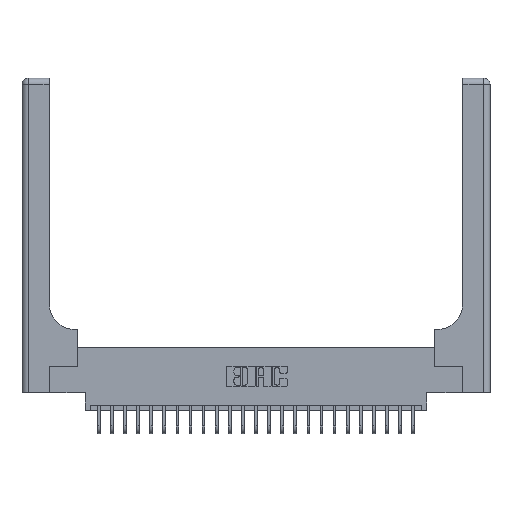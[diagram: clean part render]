
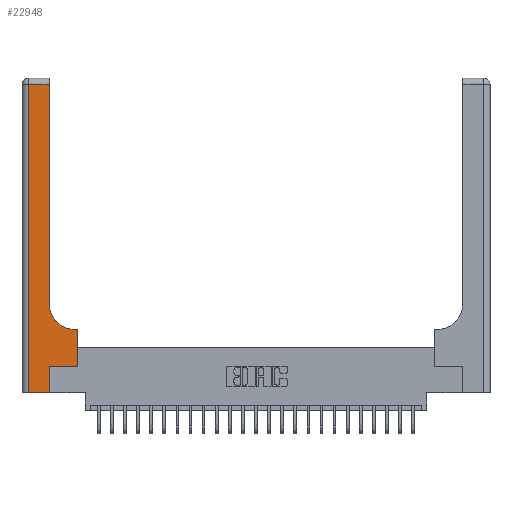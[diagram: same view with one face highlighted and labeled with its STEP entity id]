
A CAD part, top view. The second image highlights one B-rep face of the part: STEP entity #22948.
In plain terms, the highlighted planar face has unit normal (0, 0, 1).
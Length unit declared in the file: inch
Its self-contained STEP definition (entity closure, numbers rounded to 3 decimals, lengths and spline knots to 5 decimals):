
#77 = LINE ( 'NONE', #7890, #7603 ) ;
#112 = VERTEX_POINT ( 'NONE', #7689 ) ;
#280 = LINE ( 'NONE', #24262, #21089 ) ;
#475 = VERTEX_POINT ( 'NONE', #2131 ) ;
#609 = EDGE_CURVE ( 'NONE', #1662, #475, #941, .T. ) ;
#678 = CARTESIAN_POINT ( 'NONE',  ( 0.265, 0., 0.37 ) ) ;
#730 = CARTESIAN_POINT ( 'NONE',  ( 0.265, 0.25, 0.37 ) ) ;
#839 = ORIENTED_EDGE ( 'NONE', *, *, #14893, .T. ) ;
#941 = LINE ( 'NONE', #4898, #4275 ) ;
#1059 = CARTESIAN_POINT ( 'NONE',  ( 0.26, 0.6, 0.37 ) ) ;
#1343 = AXIS2_PLACEMENT_3D ( 'NONE', #14839, #16431, #24529 ) ;
#1346 = CARTESIAN_POINT ( 'NONE',  ( 0.26, 3., 0.37 ) ) ;
#1662 = VERTEX_POINT ( 'NONE', #21528 ) ;
#1991 = LINE ( 'NONE', #23966, #20015 ) ;
#2131 = CARTESIAN_POINT ( 'NONE',  ( 0.06, 2.94, 0.37 ) ) ;
#2136 = VERTEX_POINT ( 'NONE', #11423 ) ;
#3370 = AXIS2_PLACEMENT_3D ( 'NONE', #18715, #4401, #20845 ) ;
#4101 = DIRECTION ( 'NONE',  ( 0., -1., 0. ) ) ;
#4275 = VECTOR ( 'NONE', #23180, 39.37008 ) ;
#4401 = DIRECTION ( 'NONE',  ( 0., 0., -1. ) ) ;
#4898 = CARTESIAN_POINT ( 'NONE',  ( 0., 2.94, 0.37 ) ) ;
#5869 = VERTEX_POINT ( 'NONE', #25117 ) ;
#6235 = EDGE_CURVE ( 'NONE', #13222, #14108, #9724, .T. ) ;
#6571 = VERTEX_POINT ( 'NONE', #7796 ) ;
#7153 = ORIENTED_EDGE ( 'NONE', *, *, #11031, .T. ) ;
#7275 = ORIENTED_EDGE ( 'NONE', *, *, #19658, .T. ) ;
#7603 = VECTOR ( 'NONE', #16080, 39.37008 ) ;
#7689 = CARTESIAN_POINT ( 'NONE',  ( 0.528, 0.6, 0.37 ) ) ;
#7796 = CARTESIAN_POINT ( 'NONE',  ( 0.26, 0.85, 0.37 ) ) ;
#7890 = CARTESIAN_POINT ( 'NONE',  ( 0., 0., 0.37 ) ) ;
#8899 = VECTOR ( 'NONE', #13922, 39.37008 ) ;
#9143 = ORIENTED_EDGE ( 'NONE', *, *, #12044, .T. ) ;
#9724 = LINE ( 'NONE', #15902, #8899 ) ;
#10054 = ORIENTED_EDGE ( 'NONE', *, *, #25425, .T. ) ;
#11031 = EDGE_CURVE ( 'NONE', #14108, #112, #1991, .T. ) ;
#11196 = VECTOR ( 'NONE', #17512, 39.37008 ) ;
#11423 = CARTESIAN_POINT ( 'NONE',  ( 0.06, 0., 0.37 ) ) ;
#12044 = EDGE_CURVE ( 'NONE', #6571, #1662, #21476, .T. ) ;
#12598 = PLANE ( 'NONE',  #3370 ) ;
#13222 = VERTEX_POINT ( 'NONE', #730 ) ;
#13922 = DIRECTION ( 'NONE',  ( 1., 0., 0. ) ) ;
#14108 = VERTEX_POINT ( 'NONE', #19644 ) ;
#14222 = CARTESIAN_POINT ( 'NONE',  ( 0.265, 0., 0.37 ) ) ;
#14839 = CARTESIAN_POINT ( 'NONE',  ( 0.51, 0.85, 0.37 ) ) ;
#14893 = EDGE_CURVE ( 'NONE', #112, #5869, #15067, .T. ) ;
#15067 = LINE ( 'NONE', #1059, #23192 ) ;
#15902 = CARTESIAN_POINT ( 'NONE',  ( 0.265, 0.25, 0.37 ) ) ;
#16080 = DIRECTION ( 'NONE',  ( 1., 0., 0. ) ) ;
#16431 = DIRECTION ( 'NONE',  ( 0., 0., -1. ) ) ;
#16818 = DIRECTION ( 'NONE',  ( 0., 1., 0. ) ) ;
#17512 = DIRECTION ( 'NONE',  ( 0., 1., 0. ) ) ;
#17757 = DIRECTION ( 'NONE',  ( 0., 1., 0. ) ) ;
#17812 = ORIENTED_EDGE ( 'NONE', *, *, #6235, .T. ) ;
#18559 = EDGE_CURVE ( 'NONE', #19293, #13222, #21060, .T. ) ;
#18585 = FACE_OUTER_BOUND ( 'NONE', #19126, .T. ) ;
#18715 = CARTESIAN_POINT ( 'NONE',  ( 0., 3., 0.37 ) ) ;
#19126 = EDGE_LOOP ( 'NONE', ( #9143, #22020, #7275, #20267, #22399, #17812, #7153, #839, #10054 ) ) ;
#19293 = VERTEX_POINT ( 'NONE', #14222 ) ;
#19644 = CARTESIAN_POINT ( 'NONE',  ( 0.528, 0.25, 0.37 ) ) ;
#19658 = EDGE_CURVE ( 'NONE', #475, #2136, #280, .T. ) ;
#20015 = VECTOR ( 'NONE', #17757, 39.37008 ) ;
#20267 = ORIENTED_EDGE ( 'NONE', *, *, #22481, .T. ) ;
#20845 = DIRECTION ( 'NONE',  ( -1., 0., 0. ) ) ;
#21040 = DIRECTION ( 'NONE',  ( -1., 0., 0. ) ) ;
#21060 = LINE ( 'NONE', #678, #24814 ) ;
#21089 = VECTOR ( 'NONE', #4101, 39.37008 ) ;
#21476 = LINE ( 'NONE', #1346, #11196 ) ;
#21528 = CARTESIAN_POINT ( 'NONE',  ( 0.26, 2.94, 0.37 ) ) ;
#22020 = ORIENTED_EDGE ( 'NONE', *, *, #609, .T. ) ;
#22399 = ORIENTED_EDGE ( 'NONE', *, *, #18559, .T. ) ;
#22481 = EDGE_CURVE ( 'NONE', #2136, #19293, #77, .T. ) ;
#22948 = ADVANCED_FACE ( 'NONE', ( #18585 ), #12598, .F. ) ;
#23180 = DIRECTION ( 'NONE',  ( -1., 0., 0. ) ) ;
#23192 = VECTOR ( 'NONE', #21040, 39.37008 ) ;
#23966 = CARTESIAN_POINT ( 'NONE',  ( 0.528, 0.25, 0.37 ) ) ;
#24262 = CARTESIAN_POINT ( 'NONE',  ( 0.06, 3., 0.37 ) ) ;
#24529 = DIRECTION ( 'NONE',  ( 1., 0., 0. ) ) ;
#24814 = VECTOR ( 'NONE', #16818, 39.37008 ) ;
#25043 = CIRCLE ( 'NONE', #1343, 0.25 ) ;
#25117 = CARTESIAN_POINT ( 'NONE',  ( 0.51, 0.6, 0.37 ) ) ;
#25425 = EDGE_CURVE ( 'NONE', #5869, #6571, #25043, .T. ) ;
